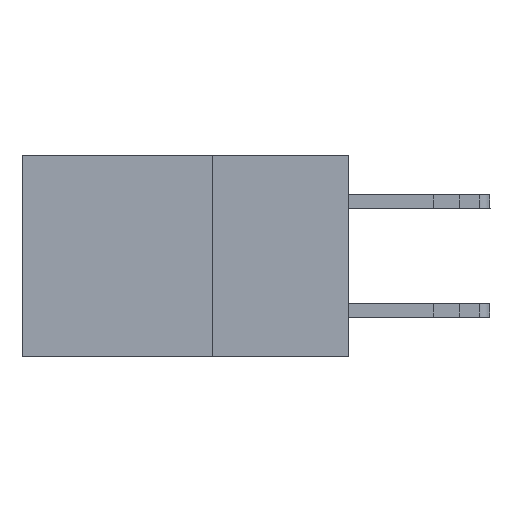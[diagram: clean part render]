
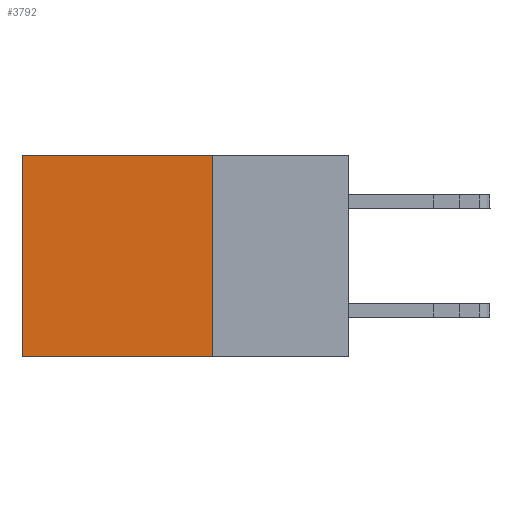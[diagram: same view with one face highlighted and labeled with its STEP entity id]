
A CAD part, left-side view. The second image highlights one B-rep face of the part: STEP entity #3792.
In plain terms, the highlighted planar face has unit normal (-1, 0, 0).
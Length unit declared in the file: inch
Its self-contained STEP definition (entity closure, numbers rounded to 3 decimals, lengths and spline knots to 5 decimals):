
#81 = VECTOR ( 'NONE', #5379, 39.37008 ) ;
#194 = CARTESIAN_POINT ( 'NONE',  ( 0.2615, 0.6, -0.37 ) ) ;
#627 = PLANE ( 'NONE',  #2923 ) ;
#638 = LINE ( 'NONE', #6796, #9333 ) ;
#1063 = VERTEX_POINT ( 'NONE', #194 ) ;
#1066 = VERTEX_POINT ( 'NONE', #4230 ) ;
#1344 = CARTESIAN_POINT ( 'NONE',  ( 0.2615, 0.6, 0. ) ) ;
#1465 = EDGE_CURVE ( 'NONE', #1066, #6240, #4013, .T. ) ;
#1513 = EDGE_CURVE ( 'NONE', #6240, #1063, #4655, .T. ) ;
#1524 = DIRECTION ( 'NONE',  ( 0., 1., 0. ) ) ;
#2194 = VERTEX_POINT ( 'NONE', #1344 ) ;
#2267 = CARTESIAN_POINT ( 'NONE',  ( 0.2615, 0.25, -0.37 ) ) ;
#2332 = DIRECTION ( 'NONE',  ( 0., 0., -1. ) ) ;
#2429 = EDGE_LOOP ( 'NONE', ( #9570, #9496, #6735, #4146 ) ) ;
#2923 = AXIS2_PLACEMENT_3D ( 'NONE', #9926, #9214, #2332 ) ;
#3322 = EDGE_CURVE ( 'NONE', #2194, #1063, #638, .T. ) ;
#3603 = CARTESIAN_POINT ( 'NONE',  ( 0.2615, 0.25, 0. ) ) ;
#3792 = ADVANCED_FACE ( 'NONE', ( #8284 ), #627, .F. ) ;
#4013 = LINE ( 'NONE', #4727, #8162 ) ;
#4146 = ORIENTED_EDGE ( 'NONE', *, *, #4826, .T. ) ;
#4230 = CARTESIAN_POINT ( 'NONE',  ( 0.2615, 0.25, 0. ) ) ;
#4348 = LINE ( 'NONE', #3603, #7206 ) ;
#4655 = LINE ( 'NONE', #2267, #81 ) ;
#4727 = CARTESIAN_POINT ( 'NONE',  ( 0.2615, 0.25, -0.37 ) ) ;
#4826 = EDGE_CURVE ( 'NONE', #1066, #2194, #4348, .T. ) ;
#5379 = DIRECTION ( 'NONE',  ( 0., 1., 0. ) ) ;
#6240 = VERTEX_POINT ( 'NONE', #8866 ) ;
#6735 = ORIENTED_EDGE ( 'NONE', *, *, #1465, .F. ) ;
#6796 = CARTESIAN_POINT ( 'NONE',  ( 0.2615, 0.6, -0.37 ) ) ;
#7000 = DIRECTION ( 'NONE',  ( 0., 0., -1. ) ) ;
#7206 = VECTOR ( 'NONE', #1524, 39.37008 ) ;
#8162 = VECTOR ( 'NONE', #7000, 39.37008 ) ;
#8284 = FACE_OUTER_BOUND ( 'NONE', #2429, .T. ) ;
#8866 = CARTESIAN_POINT ( 'NONE',  ( 0.2615, 0.25, -0.37 ) ) ;
#9214 = DIRECTION ( 'NONE',  ( 1., 0., 0. ) ) ;
#9333 = VECTOR ( 'NONE', #9894, 39.37008 ) ;
#9496 = ORIENTED_EDGE ( 'NONE', *, *, #1513, .F. ) ;
#9570 = ORIENTED_EDGE ( 'NONE', *, *, #3322, .T. ) ;
#9894 = DIRECTION ( 'NONE',  ( 0., 0., -1. ) ) ;
#9926 = CARTESIAN_POINT ( 'NONE',  ( 0.2615, 0.25, -0.37 ) ) ;
